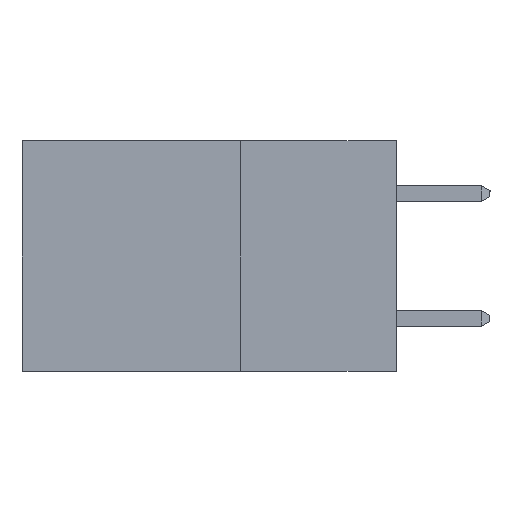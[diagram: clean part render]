
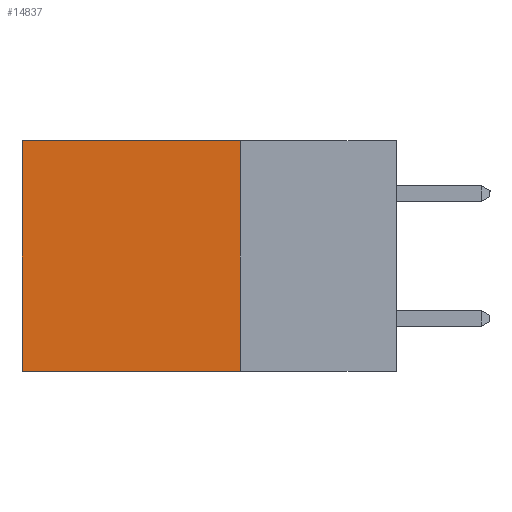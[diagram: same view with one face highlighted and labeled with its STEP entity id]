
A CAD part, left-side view. The second image highlights one B-rep face of the part: STEP entity #14837.
In plain terms, the highlighted planar face has unit normal (-1, 0, 0).
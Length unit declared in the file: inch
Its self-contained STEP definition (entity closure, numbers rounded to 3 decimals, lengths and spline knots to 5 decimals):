
#417 = VECTOR ( 'NONE', #9495, 39.37008 ) ;
#629 = VECTOR ( 'NONE', #3228, 39.37008 ) ;
#1100 = LINE ( 'NONE', #6562, #22728 ) ;
#1195 = CARTESIAN_POINT ( 'NONE',  ( 0.2615, 0.6, -0.37 ) ) ;
#1411 = DIRECTION ( 'NONE',  ( 1., 0., 0. ) ) ;
#1763 = EDGE_CURVE ( 'NONE', #6283, #8242, #1100, .T. ) ;
#1871 = PLANE ( 'NONE',  #20762 ) ;
#2637 = EDGE_CURVE ( 'NONE', #9876, #14431, #14599, .T. ) ;
#2800 = LINE ( 'NONE', #6445, #6890 ) ;
#3228 = DIRECTION ( 'NONE',  ( 0., 0., -1. ) ) ;
#4681 = DIRECTION ( 'NONE',  ( 0., 0., -1. ) ) ;
#4704 = EDGE_CURVE ( 'NONE', #6283, #9876, #2800, .T. ) ;
#6261 = ORIENTED_EDGE ( 'NONE', *, *, #2637, .F. ) ;
#6283 = VERTEX_POINT ( 'NONE', #10331 ) ;
#6445 = CARTESIAN_POINT ( 'NONE',  ( 0.2615, 0.25, -0.37 ) ) ;
#6562 = CARTESIAN_POINT ( 'NONE',  ( 0.2615, 0.25, 0. ) ) ;
#6890 = VECTOR ( 'NONE', #4681, 39.37008 ) ;
#7027 = DIRECTION ( 'NONE',  ( 0., 0., -1. ) ) ;
#8242 = VERTEX_POINT ( 'NONE', #22625 ) ;
#9495 = DIRECTION ( 'NONE',  ( 0., 1., 0. ) ) ;
#9876 = VERTEX_POINT ( 'NONE', #12846 ) ;
#10331 = CARTESIAN_POINT ( 'NONE',  ( 0.2615, 0.25, 0. ) ) ;
#10624 = LINE ( 'NONE', #16096, #629 ) ;
#11296 = CARTESIAN_POINT ( 'NONE',  ( 0.2615, 0.25, -0.37 ) ) ;
#12475 = EDGE_CURVE ( 'NONE', #8242, #14431, #10624, .T. ) ;
#12846 = CARTESIAN_POINT ( 'NONE',  ( 0.2615, 0.25, -0.37 ) ) ;
#13360 = ORIENTED_EDGE ( 'NONE', *, *, #12475, .T. ) ;
#13843 = DIRECTION ( 'NONE',  ( 0., 1., 0. ) ) ;
#14431 = VERTEX_POINT ( 'NONE', #1195 ) ;
#14479 = FACE_OUTER_BOUND ( 'NONE', #15772, .T. ) ;
#14599 = LINE ( 'NONE', #11296, #417 ) ;
#14837 = ADVANCED_FACE ( 'NONE', ( #14479 ), #1871, .F. ) ;
#15772 = EDGE_LOOP ( 'NONE', ( #13360, #6261, #23045, #19040 ) ) ;
#16096 = CARTESIAN_POINT ( 'NONE',  ( 0.2615, 0.6, -0.37 ) ) ;
#18070 = CARTESIAN_POINT ( 'NONE',  ( 0.2615, 0.25, -0.37 ) ) ;
#19040 = ORIENTED_EDGE ( 'NONE', *, *, #1763, .T. ) ;
#20762 = AXIS2_PLACEMENT_3D ( 'NONE', #18070, #1411, #7027 ) ;
#22625 = CARTESIAN_POINT ( 'NONE',  ( 0.2615, 0.6, 0. ) ) ;
#22728 = VECTOR ( 'NONE', #13843, 39.37008 ) ;
#23045 = ORIENTED_EDGE ( 'NONE', *, *, #4704, .F. ) ;
